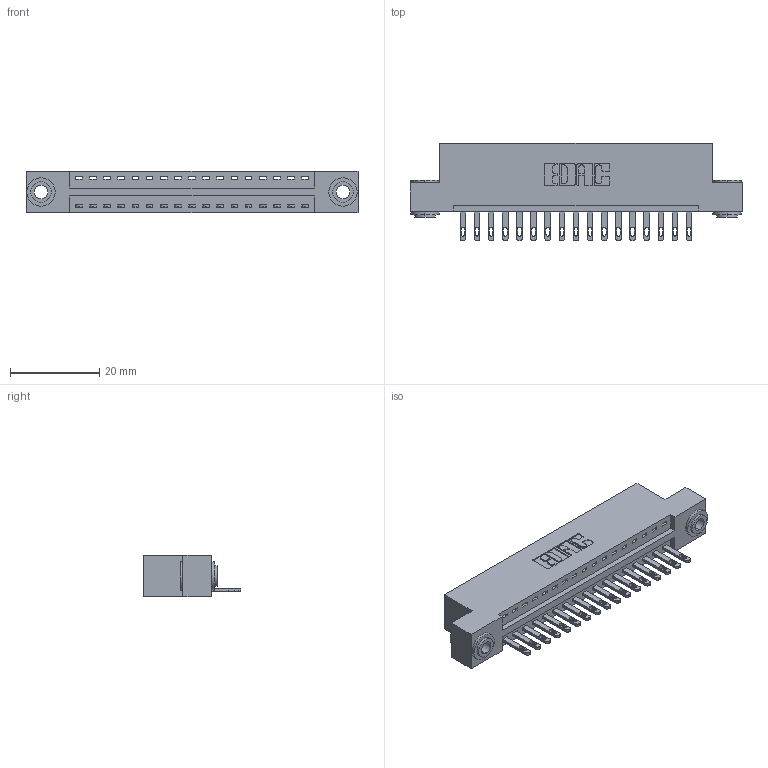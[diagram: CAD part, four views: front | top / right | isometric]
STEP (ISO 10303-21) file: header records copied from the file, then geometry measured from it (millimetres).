
FILE_DESCRIPTION (( 'STEP AP203' ), '1' );
FILE_NAME ('346-017-500-103.STEP', '2022-05-05T11:21:40', ( '' ), ( '' ), 'SwSTEP 2.0', 'SolidWorks 2020', '' );
FILE_SCHEMA (( 'CONFIG_CONTROL_DESIGN' ));
Length unit declared in the file: inch
Products named in the file (4): 345-250-002_345-250-002-102; 345-292-001_345-293-100; 346 Part_Flush Mounting Lugs - 0.156 Dia-TH; 346-017-500-103
Assembly tree (20 placements, depth 2):
  346-017-500-103
    346 Part_Flush Mounting Lugs - 0.156 Dia-TH
    345-292-001_345-293-100  x17
    345-250-002_345-250-002-102  x2
Bounding box: 74.55 x 21.84 x 9.4 mm (x, y, z)
Volume: 6975.6 mm3; surface area: 8739.9 mm2
Topology: 20 solids, 20 shells, 1092 faces, 3297 edges, 2194 vertices
Faces by surface type: plane 678, cylinder 406, cone 8
Entity records: 14912 total; most frequent: CARTESIAN_POINT 2544, ORIENTED_EDGE 2486, DIRECTION 2307, EDGE_CURVE 1243, LINE 1015, VECTOR 1015, VERTEX_POINT 826, AXIS2_PLACEMENT_3D 646
